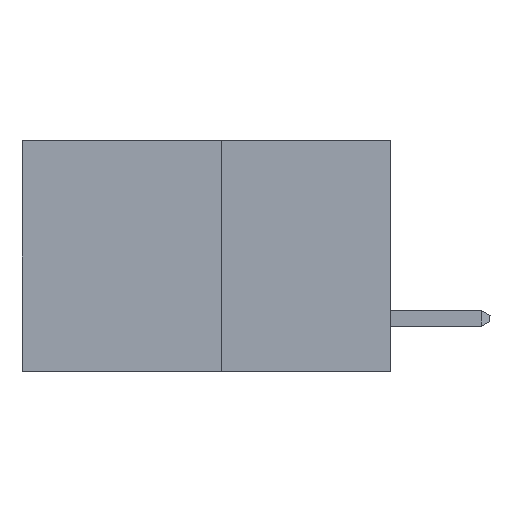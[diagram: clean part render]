
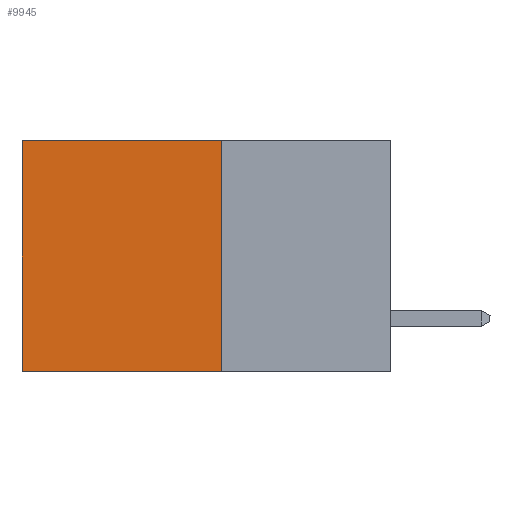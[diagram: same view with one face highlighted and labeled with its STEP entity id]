
A CAD part, left-side view. The second image highlights one B-rep face of the part: STEP entity #9945.
In plain terms, the highlighted planar face has unit normal (-1, 0, 0).
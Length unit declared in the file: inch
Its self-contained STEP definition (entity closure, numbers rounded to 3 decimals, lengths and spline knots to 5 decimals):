
#80 = ORIENTED_EDGE ( 'NONE', *, *, #13272, .T. ) ;
#585 = PLANE ( 'NONE',  #8563 ) ;
#1632 = ORIENTED_EDGE ( 'NONE', *, *, #6735, .F. ) ;
#1912 = DIRECTION ( 'NONE',  ( 0., 0., -1. ) ) ;
#2583 = VERTEX_POINT ( 'NONE', #3161 ) ;
#2800 = CARTESIAN_POINT ( 'NONE',  ( 0.277, 0.27, 0. ) ) ;
#3049 = VECTOR ( 'NONE', #9535, 39.37008 ) ;
#3144 = CARTESIAN_POINT ( 'NONE',  ( 0.277, 0.27, 0. ) ) ;
#3161 = CARTESIAN_POINT ( 'NONE',  ( 0.277, 0.59, -0.37 ) ) ;
#3812 = CARTESIAN_POINT ( 'NONE',  ( 0.277, 0.59, 0. ) ) ;
#4339 = VERTEX_POINT ( 'NONE', #3144 ) ;
#5050 = CARTESIAN_POINT ( 'NONE',  ( 0.277, 0.27, -0.37 ) ) ;
#5697 = LINE ( 'NONE', #6648, #10878 ) ;
#5803 = VECTOR ( 'NONE', #8507, 39.37008 ) ;
#5928 = ORIENTED_EDGE ( 'NONE', *, *, #10412, .F. ) ;
#6101 = VECTOR ( 'NONE', #11845, 39.37008 ) ;
#6231 = LINE ( 'NONE', #12833, #3049 ) ;
#6472 = LINE ( 'NONE', #2800, #6101 ) ;
#6482 = VERTEX_POINT ( 'NONE', #3812 ) ;
#6648 = CARTESIAN_POINT ( 'NONE',  ( 0.277, 0.27, -0.37 ) ) ;
#6735 = EDGE_CURVE ( 'NONE', #4339, #8834, #5697, .T. ) ;
#7723 = DIRECTION ( 'NONE',  ( 0., 0., -1. ) ) ;
#8252 = EDGE_CURVE ( 'NONE', #4339, #6482, #6472, .T. ) ;
#8507 = DIRECTION ( 'NONE',  ( 0., 0., -1. ) ) ;
#8563 = AXIS2_PLACEMENT_3D ( 'NONE', #9959, #8879, #1912 ) ;
#8720 = LINE ( 'NONE', #12959, #5803 ) ;
#8834 = VERTEX_POINT ( 'NONE', #5050 ) ;
#8879 = DIRECTION ( 'NONE',  ( 1., 0., 0. ) ) ;
#9535 = DIRECTION ( 'NONE',  ( 0., 1., 0. ) ) ;
#9945 = ADVANCED_FACE ( 'NONE', ( #11723 ), #585, .F. ) ;
#9959 = CARTESIAN_POINT ( 'NONE',  ( 0.277, 0.27, -0.37 ) ) ;
#10169 = EDGE_LOOP ( 'NONE', ( #80, #5928, #1632, #15046 ) ) ;
#10412 = EDGE_CURVE ( 'NONE', #8834, #2583, #6231, .T. ) ;
#10878 = VECTOR ( 'NONE', #7723, 39.37008 ) ;
#11723 = FACE_OUTER_BOUND ( 'NONE', #10169, .T. ) ;
#11845 = DIRECTION ( 'NONE',  ( 0., 1., 0. ) ) ;
#12833 = CARTESIAN_POINT ( 'NONE',  ( 0.277, 0.27, -0.37 ) ) ;
#12959 = CARTESIAN_POINT ( 'NONE',  ( 0.277, 0.59, -0.37 ) ) ;
#13272 = EDGE_CURVE ( 'NONE', #6482, #2583, #8720, .T. ) ;
#15046 = ORIENTED_EDGE ( 'NONE', *, *, #8252, .T. ) ;
